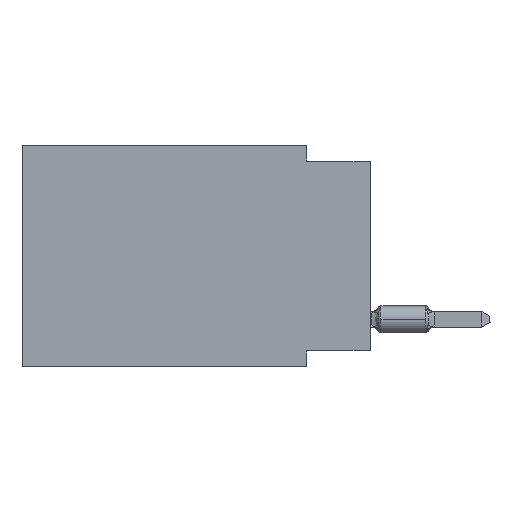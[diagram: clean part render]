
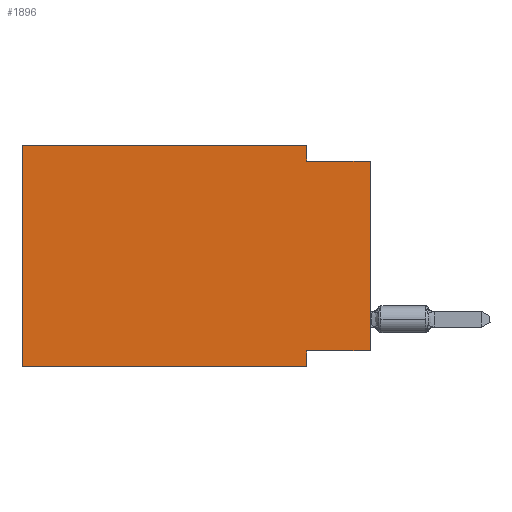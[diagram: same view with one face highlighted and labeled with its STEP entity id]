
A CAD part, left-side view. The second image highlights one B-rep face of the part: STEP entity #1896.
In plain terms, the highlighted planar face has unit normal (-1, 0, 0).
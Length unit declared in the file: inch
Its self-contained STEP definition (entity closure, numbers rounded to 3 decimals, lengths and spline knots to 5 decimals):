
#13 = EDGE_CURVE ( 'NONE', #28223, #19430, #25132, .T. ) ;
#1896 = ADVANCED_FACE ( 'NONE', ( #16121 ), #24613, .F. ) ;
#3300 = LINE ( 'NONE', #18046, #19781 ) ;
#4189 = VECTOR ( 'NONE', #31692, 39.37008 ) ;
#4408 = CARTESIAN_POINT ( 'NONE',  ( 0., 0.1, 0. ) ) ;
#4813 = DIRECTION ( 'NONE',  ( 0., 0., -1. ) ) ;
#5023 = CARTESIAN_POINT ( 'NONE',  ( 0., 0.1, -0.35 ) ) ;
#5546 = VERTEX_POINT ( 'NONE', #5023 ) ;
#5590 = LINE ( 'NONE', #34604, #26516 ) ;
#6182 = CARTESIAN_POINT ( 'NONE',  ( 0., 0.55, -0.35 ) ) ;
#8176 = VECTOR ( 'NONE', #36318, 39.37008 ) ;
#8966 = ORIENTED_EDGE ( 'NONE', *, *, #19656, .F. ) ;
#9641 = EDGE_LOOP ( 'NONE', ( #21287, #12884, #23423, #31385, #8966, #10215, #16086, #17507 ) ) ;
#10215 = ORIENTED_EDGE ( 'NONE', *, *, #16621, .T. ) ;
#11233 = CARTESIAN_POINT ( 'NONE',  ( 0., 0., -0.025 ) ) ;
#11636 = EDGE_CURVE ( 'NONE', #26028, #28223, #18173, .T. ) ;
#12640 = DIRECTION ( 'NONE',  ( 0., -1., 0. ) ) ;
#12884 = ORIENTED_EDGE ( 'NONE', *, *, #23967, .F. ) ;
#13056 = DIRECTION ( 'NONE',  ( 1., 0., 0. ) ) ;
#15352 = EDGE_CURVE ( 'NONE', #15725, #5546, #30461, .T. ) ;
#15725 = VERTEX_POINT ( 'NONE', #26378 ) ;
#16086 = ORIENTED_EDGE ( 'NONE', *, *, #15352, .F. ) ;
#16121 = FACE_OUTER_BOUND ( 'NONE', #9641, .T. ) ;
#16168 = CARTESIAN_POINT ( 'NONE',  ( 0., 0.55, 0. ) ) ;
#16213 = DIRECTION ( 'NONE',  ( 0., 0., 1. ) ) ;
#16241 = CARTESIAN_POINT ( 'NONE',  ( 0., 0.1, -0.025 ) ) ;
#16389 = CARTESIAN_POINT ( 'NONE',  ( 0., 0.1, -0.35 ) ) ;
#16621 = EDGE_CURVE ( 'NONE', #26733, #5546, #3300, .T. ) ;
#16794 = CARTESIAN_POINT ( 'NONE',  ( 0., 0., -0.325 ) ) ;
#17075 = CARTESIAN_POINT ( 'NONE',  ( 0., 0., -0.325 ) ) ;
#17507 = ORIENTED_EDGE ( 'NONE', *, *, #22199, .F. ) ;
#18046 = CARTESIAN_POINT ( 'NONE',  ( 0., 0.55, -0.35 ) ) ;
#18173 = LINE ( 'NONE', #29912, #27104 ) ;
#19430 = VERTEX_POINT ( 'NONE', #16241 ) ;
#19550 = VECTOR ( 'NONE', #16213, 39.37008 ) ;
#19656 = EDGE_CURVE ( 'NONE', #26733, #26028, #5590, .T. ) ;
#19781 = VECTOR ( 'NONE', #35481, 39.37008 ) ;
#20030 = VERTEX_POINT ( 'NONE', #11233 ) ;
#20112 = DIRECTION ( 'NONE',  ( 0., -1., 0. ) ) ;
#20283 = VECTOR ( 'NONE', #36727, 39.37008 ) ;
#20518 = VECTOR ( 'NONE', #20112, 39.37008 ) ;
#21287 = ORIENTED_EDGE ( 'NONE', *, *, #32357, .T. ) ;
#22199 = EDGE_CURVE ( 'NONE', #23774, #15725, #23843, .T. ) ;
#23423 = ORIENTED_EDGE ( 'NONE', *, *, #13, .F. ) ;
#23774 = VERTEX_POINT ( 'NONE', #17075 ) ;
#23843 = LINE ( 'NONE', #16794, #20283 ) ;
#23967 = EDGE_CURVE ( 'NONE', #19430, #20030, #28118, .T. ) ;
#24613 = PLANE ( 'NONE',  #30863 ) ;
#25132 = LINE ( 'NONE', #31574, #4189 ) ;
#26028 = VERTEX_POINT ( 'NONE', #34132 ) ;
#26378 = CARTESIAN_POINT ( 'NONE',  ( 0., 0.1, -0.325 ) ) ;
#26516 = VECTOR ( 'NONE', #34716, 39.37008 ) ;
#26733 = VERTEX_POINT ( 'NONE', #6182 ) ;
#27104 = VECTOR ( 'NONE', #12640, 39.37008 ) ;
#28118 = LINE ( 'NONE', #30474, #20518 ) ;
#28223 = VERTEX_POINT ( 'NONE', #4408 ) ;
#29912 = CARTESIAN_POINT ( 'NONE',  ( 0., 0.55, 0. ) ) ;
#30143 = CARTESIAN_POINT ( 'NONE',  ( 0., 0., 0. ) ) ;
#30461 = LINE ( 'NONE', #16389, #8176 ) ;
#30474 = CARTESIAN_POINT ( 'NONE',  ( 0., 0., -0.025 ) ) ;
#30863 = AXIS2_PLACEMENT_3D ( 'NONE', #16168, #13056, #4813 ) ;
#31385 = ORIENTED_EDGE ( 'NONE', *, *, #11636, .F. ) ;
#31574 = CARTESIAN_POINT ( 'NONE',  ( 0., 0.1, 0. ) ) ;
#31692 = DIRECTION ( 'NONE',  ( 0., 0., -1. ) ) ;
#32357 = EDGE_CURVE ( 'NONE', #23774, #20030, #35133, .T. ) ;
#34132 = CARTESIAN_POINT ( 'NONE',  ( 0., 0.55, 0. ) ) ;
#34604 = CARTESIAN_POINT ( 'NONE',  ( 0., 0.55, 0. ) ) ;
#34716 = DIRECTION ( 'NONE',  ( 0., 0., 1. ) ) ;
#35133 = LINE ( 'NONE', #30143, #19550 ) ;
#35481 = DIRECTION ( 'NONE',  ( 0., -1., 0. ) ) ;
#36318 = DIRECTION ( 'NONE',  ( 0., 0., -1. ) ) ;
#36727 = DIRECTION ( 'NONE',  ( 0., 1., 0. ) ) ;
